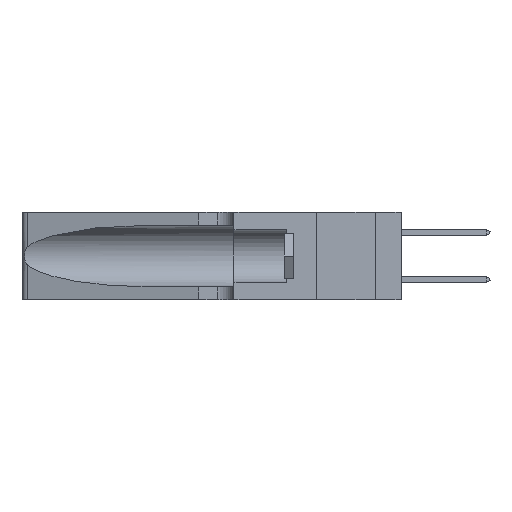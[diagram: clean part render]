
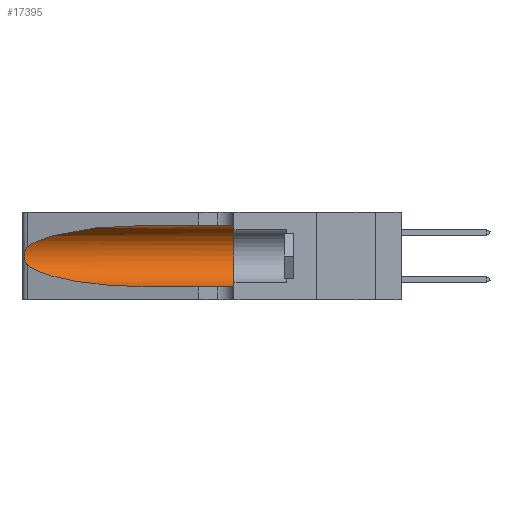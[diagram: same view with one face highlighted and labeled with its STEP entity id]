
A CAD part, left-side view. The second image highlights one B-rep face of the part: STEP entity #17395.
In plain terms, the highlighted cylindrical face has radius 3.308 mm (diameter 6.617 mm), a partial arc.
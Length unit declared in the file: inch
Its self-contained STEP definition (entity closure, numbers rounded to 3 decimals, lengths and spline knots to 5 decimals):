
#262 = DIRECTION ( 'NONE',  ( 0., -1., 0. ) ) ;
#572 =( BOUNDED_CURVE ( )  B_SPLINE_CURVE ( 3, ( #20406, #8138, #22127, #11738 ),
 .UNSPECIFIED., .F., .T. ) 
 B_SPLINE_CURVE_WITH_KNOTS ( ( 4, 4 ),
 ( 3.44316, 4.71239 ),
 .UNSPECIFIED. ) 
 CURVE ( )  GEOMETRIC_REPRESENTATION_ITEM ( )  RATIONAL_B_SPLINE_CURVE ( ( 1., 0.87, 0.87, 1. ) ) 
 REPRESENTATION_ITEM ( '' )  );
#617 = CARTESIAN_POINT ( 'NONE',  ( 0.25639, 1.23186, 0.15144 ) ) ;
#1048 = LINE ( 'NONE', #15624, #5889 ) ;
#1193 = ORIENTED_EDGE ( 'NONE', *, *, #10845, .T. ) ;
#1351 = CARTESIAN_POINT ( 'NONE',  ( 0.18966, 0.96281, 0.31525 ) ) ;
#1633 =( BOUNDED_CURVE ( )  B_SPLINE_CURVE ( 3, ( #17276, #1351, #15608, #5020 ),
 .UNSPECIFIED., .F., .F. ) 
 B_SPLINE_CURVE_WITH_KNOTS ( ( 4, 4 ),
 ( 1.5708, 2.84003 ),
 .UNSPECIFIED. ) 
 CURVE ( )  GEOMETRIC_REPRESENTATION_ITEM ( )  RATIONAL_B_SPLINE_CURVE ( ( 1., 0.87, 0.87, 1. ) ) 
 REPRESENTATION_ITEM ( '' )  );
#1634 = B_SPLINE_CURVE_WITH_KNOTS ( 'NONE', 3,
 ( #5794, #5863, #4248, #16584, #6029, #18337, #7807, #20073, #9621, #21810, #11401, #617, #13171, #2471 ),
 .UNSPECIFIED., .F., .F.,
 ( 4, 2, 2, 2, 2, 2, 4 ),
 ( 0., 0.00027, 0.00053, 0.00107, 0.0016, 0.00187, 0.00214 ),
 .UNSPECIFIED. ) ;
#2471 = CARTESIAN_POINT ( 'NONE',  ( 0.25487, 1.22718, 0.14631 ) ) ;
#3707 = CARTESIAN_POINT ( 'NONE',  ( 0.1305, 0.72297, 0.31525 ) ) ;
#3856 = ORIENTED_EDGE ( 'NONE', *, *, #7724, .T. ) ;
#4248 = CARTESIAN_POINT ( 'NONE',  ( 0.25639, 1.23184, 0.21858 ) ) ;
#4887 = DIRECTION ( 'NONE',  ( 0., -1., 0. ) ) ;
#5020 = CARTESIAN_POINT ( 'NONE',  ( 0.25487, 1.22718, 0.22369 ) ) ;
#5040 = DIRECTION ( 'NONE',  ( 0., -1., 0. ) ) ;
#5438 = ORIENTED_EDGE ( 'NONE', *, *, #7458, .T. ) ;
#5794 = CARTESIAN_POINT ( 'NONE',  ( 0.25487, 1.22718, 0.22369 ) ) ;
#5863 = CARTESIAN_POINT ( 'NONE',  ( 0.25555, 1.22994, 0.2215 ) ) ;
#5889 = VECTOR ( 'NONE', #5040, 39.37008 ) ;
#6029 = CARTESIAN_POINT ( 'NONE',  ( 0.25854, 1.2359, 0.20912 ) ) ;
#6090 = EDGE_CURVE ( 'NONE', #11048, #16993, #15073, .T. ) ;
#6897 = CARTESIAN_POINT ( 'NONE',  ( 0.1305, 0.35, 0.185 ) ) ;
#7453 = ORIENTED_EDGE ( 'NONE', *, *, #19119, .T. ) ;
#7458 = EDGE_CURVE ( 'NONE', #15824, #18169, #1634, .T. ) ;
#7724 = EDGE_CURVE ( 'NONE', #11048, #15824, #1633, .T. ) ;
#7807 = CARTESIAN_POINT ( 'NONE',  ( 0.26075, 1.23896, 0.19203 ) ) ;
#8138 = CARTESIAN_POINT ( 'NONE',  ( 0.2373, 1.15595, 0.08982 ) ) ;
#8683 = DIRECTION ( 'NONE',  ( 0., 0., 1. ) ) ;
#9390 = ORIENTED_EDGE ( 'NONE', *, *, #10903, .F. ) ;
#9621 = CARTESIAN_POINT ( 'NONE',  ( 0.26017, 1.23833, 0.17102 ) ) ;
#9992 = CARTESIAN_POINT ( 'NONE',  ( 0.1305, 0.35, 0.05475 ) ) ;
#10845 = EDGE_CURVE ( 'NONE', #17034, #15775, #1048, .T. ) ;
#10903 = EDGE_CURVE ( 'NONE', #16993, #15775, #18821, .T. ) ;
#11048 = VERTEX_POINT ( 'NONE', #3707 ) ;
#11401 = CARTESIAN_POINT ( 'NONE',  ( 0.25789, 1.23486, 0.15765 ) ) ;
#11670 = EDGE_LOOP ( 'NONE', ( #3856, #5438, #7453, #1193, #9390, #22113 ) ) ;
#11738 = CARTESIAN_POINT ( 'NONE',  ( 0.1305, 0.72297, 0.05475 ) ) ;
#13171 = CARTESIAN_POINT ( 'NONE',  ( 0.25555, 1.22993, 0.14849 ) ) ;
#13979 = VECTOR ( 'NONE', #262, 39.37008 ) ;
#14510 = CARTESIAN_POINT ( 'NONE',  ( 0.1305, 0.35, 0.31525 ) ) ;
#14522 = CARTESIAN_POINT ( 'NONE',  ( 0.1305, 1.61858, 0.31525 ) ) ;
#15067 = CYLINDRICAL_SURFACE ( 'NONE', #22163, 0.13025 ) ;
#15073 = LINE ( 'NONE', #14522, #13979 ) ;
#15476 = CARTESIAN_POINT ( 'NONE',  ( 0.1305, 1.61858, 0.185 ) ) ;
#15608 = CARTESIAN_POINT ( 'NONE',  ( 0.2373, 1.15595, 0.28018 ) ) ;
#15616 = FACE_OUTER_BOUND ( 'NONE', #11670, .T. ) ;
#15624 = CARTESIAN_POINT ( 'NONE',  ( 0.1305, 1.61858, 0.05475 ) ) ;
#15775 = VERTEX_POINT ( 'NONE', #9992 ) ;
#15824 = VERTEX_POINT ( 'NONE', #18773 ) ;
#16584 = CARTESIAN_POINT ( 'NONE',  ( 0.25787, 1.23484, 0.2124 ) ) ;
#16993 = VERTEX_POINT ( 'NONE', #14510 ) ;
#17034 = VERTEX_POINT ( 'NONE', #18004 ) ;
#17216 = DIRECTION ( 'NONE',  ( 0., 0., -1. ) ) ;
#17276 = CARTESIAN_POINT ( 'NONE',  ( 0.1305, 0.72297, 0.31525 ) ) ;
#17395 = ADVANCED_FACE ( 'NONE', ( #15616 ), #15067, .F. ) ;
#18004 = CARTESIAN_POINT ( 'NONE',  ( 0.1305, 0.72297, 0.05475 ) ) ;
#18169 = VERTEX_POINT ( 'NONE', #19627 ) ;
#18337 = CARTESIAN_POINT ( 'NONE',  ( 0.26018, 1.23835, 0.19895 ) ) ;
#18773 = CARTESIAN_POINT ( 'NONE',  ( 0.25487, 1.22718, 0.22369 ) ) ;
#18821 = CIRCLE ( 'NONE', #19546, 0.13025 ) ;
#19119 = EDGE_CURVE ( 'NONE', #18169, #17034, #572, .T. ) ;
#19198 = DIRECTION ( 'NONE',  ( 0., 1., 0. ) ) ;
#19546 = AXIS2_PLACEMENT_3D ( 'NONE', #6897, #19198, #8683 ) ;
#19627 = CARTESIAN_POINT ( 'NONE',  ( 0.25487, 1.22718, 0.14631 ) ) ;
#20073 = CARTESIAN_POINT ( 'NONE',  ( 0.26075, 1.23896, 0.178 ) ) ;
#20406 = CARTESIAN_POINT ( 'NONE',  ( 0.25487, 1.22718, 0.14631 ) ) ;
#21810 = CARTESIAN_POINT ( 'NONE',  ( 0.25856, 1.23593, 0.16098 ) ) ;
#22113 = ORIENTED_EDGE ( 'NONE', *, *, #6090, .F. ) ;
#22127 = CARTESIAN_POINT ( 'NONE',  ( 0.18966, 0.96281, 0.05475 ) ) ;
#22163 = AXIS2_PLACEMENT_3D ( 'NONE', #15476, #4887, #17216 ) ;
